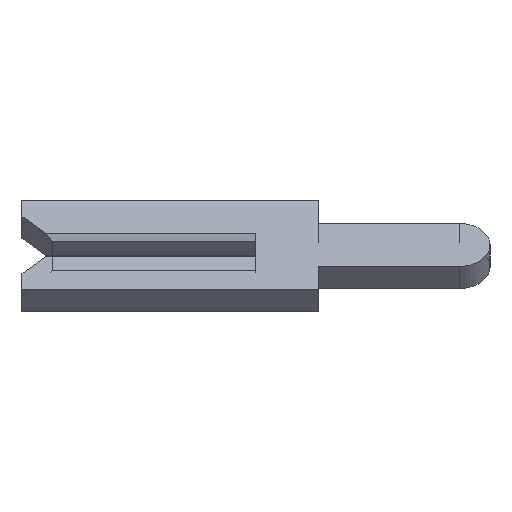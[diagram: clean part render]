
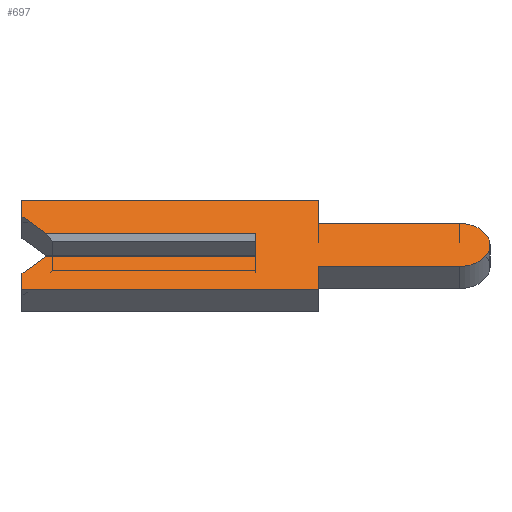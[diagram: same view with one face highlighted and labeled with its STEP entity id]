
A CAD part, left-side view. The second image highlights one B-rep face of the part: STEP entity #697.
In plain terms, the highlighted face is planar.
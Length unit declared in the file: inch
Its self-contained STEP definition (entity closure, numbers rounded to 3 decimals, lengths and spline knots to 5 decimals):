
#10 = DIRECTION ( 'NONE',  ( 0., -1., 0. ) ) ;
#16 = CARTESIAN_POINT ( 'NONE',  ( -0.01, -0.04, -0.04 ) ) ;
#23 = CARTESIAN_POINT ( 'NONE',  ( -0.01, 0.15, -0.026 ) ) ;
#36 = DIRECTION ( 'NONE',  ( 0., 0., 1. ) ) ;
#42 = DIRECTION ( 'NONE',  ( 0., 0., -1. ) ) ;
#60 = ORIENTED_EDGE ( 'NONE', *, *, #1767, .F. ) ;
#63 = DIRECTION ( 'NONE',  ( 0., -0.707, 0.707 ) ) ;
#119 = ORIENTED_EDGE ( 'NONE', *, *, #522, .F. ) ;
#129 = VECTOR ( 'NONE', #787, 39.37008 ) ;
#131 = CARTESIAN_POINT ( 'NONE',  ( -0.01, -0.04, 0.0195 ) ) ;
#186 = LINE ( 'NONE', #1748, #1643 ) ;
#199 = DIRECTION ( 'NONE',  ( 1., 0., 0. ) ) ;
#218 = VERTEX_POINT ( 'NONE', #873 ) ;
#220 = CARTESIAN_POINT ( 'NONE',  ( -0.01, -0.1305, -0.01 ) ) ;
#235 = VERTEX_POINT ( 'NONE', #1595 ) ;
#254 = EDGE_CURVE ( 'NONE', #751, #1105, #316, .T. ) ;
#256 = ORIENTED_EDGE ( 'NONE', *, *, #1512, .F. ) ;
#266 = DIRECTION ( 'NONE',  ( 0., 0., -1. ) ) ;
#316 = LINE ( 'NONE', #1175, #985 ) ;
#320 = EDGE_CURVE ( 'NONE', #235, #1173, #435, .T. ) ;
#350 = ORIENTED_EDGE ( 'NONE', *, *, #1382, .F. ) ;
#353 = VERTEX_POINT ( 'NONE', #16 ) ;
#411 = LINE ( 'NONE', #665, #1071 ) ;
#435 = LINE ( 'NONE', #23, #1765 ) ;
#454 = ORIENTED_EDGE ( 'NONE', *, *, #1727, .F. ) ;
#522 = EDGE_CURVE ( 'NONE', #706, #353, #1352, .T. ) ;
#523 = VECTOR ( 'NONE', #573, 39.37008 ) ;
#530 = VECTOR ( 'NONE', #774, 39.37008 ) ;
#533 = CARTESIAN_POINT ( 'NONE',  ( -0.01, 0.1305, 0.0065 ) ) ;
#540 = LINE ( 'NONE', #1666, #1670 ) ;
#561 = CARTESIAN_POINT ( 'NONE',  ( -0.01, 0.134, -0.01 ) ) ;
#573 = DIRECTION ( 'NONE',  ( 0., -1., 0. ) ) ;
#599 = AXIS2_PLACEMENT_3D ( 'NONE', #1445, #1133, #266 ) ;
#641 = LINE ( 'NONE', #131, #1772 ) ;
#656 = CARTESIAN_POINT ( 'NONE',  ( -0.01, -0.04, 0.0195 ) ) ;
#665 = CARTESIAN_POINT ( 'NONE',  ( -0.01, 0.15, 0.026 ) ) ;
#671 = DIRECTION ( 'NONE',  ( 0., 0., -1. ) ) ;
#695 = VECTOR ( 'NONE', #63, 39.37008 ) ;
#697 = ADVANCED_FACE ( 'NONE', ( #1655 ), #1614, .F. ) ;
#706 = VERTEX_POINT ( 'NONE', #764 ) ;
#749 = CARTESIAN_POINT ( 'NONE',  ( -0.01, -0.1305, 0. ) ) ;
#751 = VERTEX_POINT ( 'NONE', #1750 ) ;
#764 = CARTESIAN_POINT ( 'NONE',  ( -0.01, -0.04, -0.0195 ) ) ;
#774 = DIRECTION ( 'NONE',  ( 0., 0., -1. ) ) ;
#787 = DIRECTION ( 'NONE',  ( 0., -1., 0. ) ) ;
#806 = CARTESIAN_POINT ( 'NONE',  ( -0.01, -0.04, 0.04 ) ) ;
#837 = VERTEX_POINT ( 'NONE', #894 ) ;
#858 = ORIENTED_EDGE ( 'NONE', *, *, #1644, .T. ) ;
#860 = CARTESIAN_POINT ( 'NONE',  ( -0.01, -0.04, -0.04 ) ) ;
#862 = VERTEX_POINT ( 'NONE', #1333 ) ;
#873 = CARTESIAN_POINT ( 'NONE',  ( -0.01, 0., 0.01 ) ) ;
#894 = CARTESIAN_POINT ( 'NONE',  ( -0.01, -0.1305, 0.0195 ) ) ;
#917 = AXIS2_PLACEMENT_3D ( 'NONE', #749, #199, #42 ) ;
#926 = CARTESIAN_POINT ( 'NONE',  ( -0.01, 0.15, -0.026 ) ) ;
#929 = ORIENTED_EDGE ( 'NONE', *, *, #1356, .F. ) ;
#950 = VERTEX_POINT ( 'NONE', #1756 ) ;
#969 = CIRCLE ( 'NONE', #599, 0.0195 ) ;
#972 = CARTESIAN_POINT ( 'NONE',  ( -0.01, -0.04, 0.04 ) ) ;
#985 = VECTOR ( 'NONE', #10, 39.37008 ) ;
#987 = CARTESIAN_POINT ( 'NONE',  ( -0.01, 0., -0.01 ) ) ;
#991 = EDGE_CURVE ( 'NONE', #1173, #1665, #1651, .T. ) ;
#1018 = DIRECTION ( 'NONE',  ( 0., 0., 1. ) ) ;
#1030 = EDGE_CURVE ( 'NONE', #1665, #1541, #1700, .T. ) ;
#1059 = VECTOR ( 'NONE', #671, 39.37008 ) ;
#1071 = VECTOR ( 'NONE', #1505, 39.37008 ) ;
#1082 = VERTEX_POINT ( 'NONE', #656 ) ;
#1094 = DIRECTION ( 'NONE',  ( 0., 1., 0. ) ) ;
#1105 = VERTEX_POINT ( 'NONE', #806 ) ;
#1121 = LINE ( 'NONE', #972, #1059 ) ;
#1124 = ORIENTED_EDGE ( 'NONE', *, *, #1418, .F. ) ;
#1133 = DIRECTION ( 'NONE',  ( 1., 0., 0. ) ) ;
#1155 = EDGE_CURVE ( 'NONE', #1757, #751, #411, .T. ) ;
#1173 = VERTEX_POINT ( 'NONE', #926 ) ;
#1175 = CARTESIAN_POINT ( 'NONE',  ( -0.01, 0.15, 0.04 ) ) ;
#1176 = ORIENTED_EDGE ( 'NONE', *, *, #254, .F. ) ;
#1250 = DIRECTION ( 'NONE',  ( 0., 0.707, 0.707 ) ) ;
#1277 = CARTESIAN_POINT ( 'NONE',  ( -0.01, 0.15, 0.026 ) ) ;
#1296 = ORIENTED_EDGE ( 'NONE', *, *, #320, .F. ) ;
#1333 = CARTESIAN_POINT ( 'NONE',  ( -0.01, 0.134, 0.01 ) ) ;
#1347 = CARTESIAN_POINT ( 'NONE',  ( -0.01, 0.1305, -0.0065 ) ) ;
#1352 = LINE ( 'NONE', #860, #530 ) ;
#1356 = EDGE_CURVE ( 'NONE', #862, #1757, #1404, .T. ) ;
#1382 = EDGE_CURVE ( 'NONE', #1105, #1082, #1121, .T. ) ;
#1404 = LINE ( 'NONE', #533, #1604 ) ;
#1418 = EDGE_CURVE ( 'NONE', #353, #235, #540, .T. ) ;
#1422 = CARTESIAN_POINT ( 'NONE',  ( -0.01, 0.15, 0.01 ) ) ;
#1445 = CARTESIAN_POINT ( 'NONE',  ( -0.01, -0.1305, 0. ) ) ;
#1451 = ORIENTED_EDGE ( 'NONE', *, *, #991, .F. ) ;
#1468 = LINE ( 'NONE', #1695, #1781 ) ;
#1505 = DIRECTION ( 'NONE',  ( 0., 0., 1. ) ) ;
#1512 = EDGE_CURVE ( 'NONE', #950, #706, #1468, .T. ) ;
#1541 = VERTEX_POINT ( 'NONE', #987 ) ;
#1545 = DIRECTION ( 'NONE',  ( 0., 1., 0. ) ) ;
#1547 = EDGE_CURVE ( 'NONE', #837, #950, #969, .T. ) ;
#1561 = EDGE_LOOP ( 'NONE', ( #858, #60, #1627, #1451, #1296, #1124, #119, #256, #1584, #454, #350, #1176, #1760, #929 ) ) ;
#1568 = DIRECTION ( 'NONE',  ( 0., -1., 0. ) ) ;
#1584 = ORIENTED_EDGE ( 'NONE', *, *, #1547, .F. ) ;
#1595 = CARTESIAN_POINT ( 'NONE',  ( -0.01, 0.15, -0.04 ) ) ;
#1604 = VECTOR ( 'NONE', #1250, 39.37008 ) ;
#1614 = PLANE ( 'NONE',  #917 ) ;
#1627 = ORIENTED_EDGE ( 'NONE', *, *, #1030, .F. ) ;
#1643 = VECTOR ( 'NONE', #36, 39.37008 ) ;
#1644 = EDGE_CURVE ( 'NONE', #862, #218, #1697, .T. ) ;
#1651 = LINE ( 'NONE', #1347, #695 ) ;
#1655 = FACE_OUTER_BOUND ( 'NONE', #1561, .T. ) ;
#1665 = VERTEX_POINT ( 'NONE', #561 ) ;
#1666 = CARTESIAN_POINT ( 'NONE',  ( -0.01, 0.15, -0.04 ) ) ;
#1670 = VECTOR ( 'NONE', #1545, 39.37008 ) ;
#1695 = CARTESIAN_POINT ( 'NONE',  ( -0.01, -0.04, -0.0195 ) ) ;
#1697 = LINE ( 'NONE', #1422, #523 ) ;
#1700 = LINE ( 'NONE', #220, #129 ) ;
#1727 = EDGE_CURVE ( 'NONE', #1082, #837, #641, .T. ) ;
#1748 = CARTESIAN_POINT ( 'NONE',  ( -0.01, 0., 0.0065 ) ) ;
#1750 = CARTESIAN_POINT ( 'NONE',  ( -0.01, 0.15, 0.04 ) ) ;
#1756 = CARTESIAN_POINT ( 'NONE',  ( -0.01, -0.1305, -0.0195 ) ) ;
#1757 = VERTEX_POINT ( 'NONE', #1277 ) ;
#1760 = ORIENTED_EDGE ( 'NONE', *, *, #1155, .F. ) ;
#1765 = VECTOR ( 'NONE', #1018, 39.37008 ) ;
#1767 = EDGE_CURVE ( 'NONE', #1541, #218, #186, .T. ) ;
#1772 = VECTOR ( 'NONE', #1568, 39.37008 ) ;
#1781 = VECTOR ( 'NONE', #1094, 39.37008 ) ;
